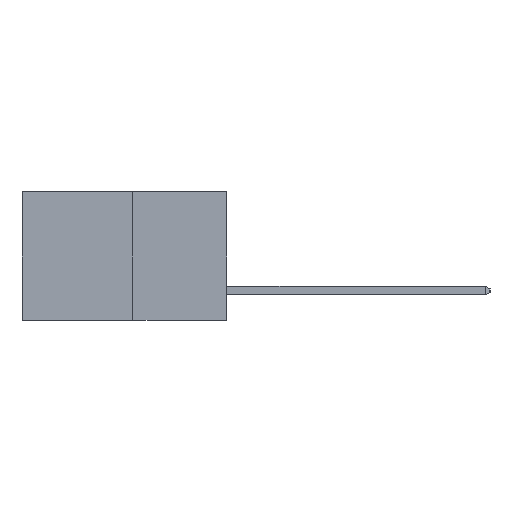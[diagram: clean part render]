
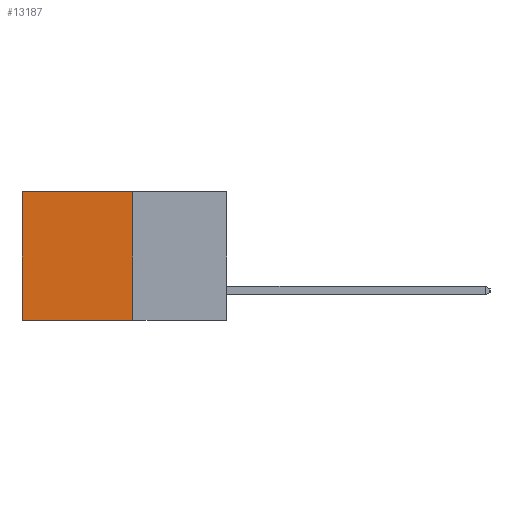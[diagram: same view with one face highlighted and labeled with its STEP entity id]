
A CAD part, left-side view. The second image highlights one B-rep face of the part: STEP entity #13187.
In plain terms, the highlighted planar face has unit normal (-1, 0, 0).
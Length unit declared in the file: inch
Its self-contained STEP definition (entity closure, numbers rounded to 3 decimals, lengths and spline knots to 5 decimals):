
#35 = CARTESIAN_POINT ( 'NONE',  ( 0.277, 0.27, -0.37 ) ) ;
#270 = PLANE ( 'NONE',  #1270 ) ;
#293 = CARTESIAN_POINT ( 'NONE',  ( 0.277, 0.59, -0.37 ) ) ;
#1270 = AXIS2_PLACEMENT_3D ( 'NONE', #7838, #8938, #2508 ) ;
#1668 = EDGE_CURVE ( 'NONE', #4268, #11095, #5689, .T. ) ;
#1980 = DIRECTION ( 'NONE',  ( 0., 1., 0. ) ) ;
#2292 = ORIENTED_EDGE ( 'NONE', *, *, #5772, .F. ) ;
#2508 = DIRECTION ( 'NONE',  ( 0., 0., -1. ) ) ;
#2675 = VECTOR ( 'NONE', #1980, 39.37008 ) ;
#3080 = DIRECTION ( 'NONE',  ( 0., 0., -1. ) ) ;
#3227 = CARTESIAN_POINT ( 'NONE',  ( 0.277, 0.27, 0. ) ) ;
#3322 = CARTESIAN_POINT ( 'NONE',  ( 0.277, 0.27, -0.37 ) ) ;
#3680 = ORIENTED_EDGE ( 'NONE', *, *, #12041, .T. ) ;
#3833 = EDGE_CURVE ( 'NONE', #4268, #5581, #13016, .T. ) ;
#4268 = VERTEX_POINT ( 'NONE', #3227 ) ;
#5500 = LINE ( 'NONE', #35, #2675 ) ;
#5581 = VERTEX_POINT ( 'NONE', #3322 ) ;
#5689 = LINE ( 'NONE', #11578, #8559 ) ;
#5772 = EDGE_CURVE ( 'NONE', #5581, #10392, #5500, .T. ) ;
#5803 = EDGE_LOOP ( 'NONE', ( #3680, #2292, #6665, #10398 ) ) ;
#6665 = ORIENTED_EDGE ( 'NONE', *, *, #3833, .F. ) ;
#7242 = VECTOR ( 'NONE', #11747, 39.37008 ) ;
#7838 = CARTESIAN_POINT ( 'NONE',  ( 0.277, 0.27, -0.37 ) ) ;
#8093 = VECTOR ( 'NONE', #3080, 39.37008 ) ;
#8444 = LINE ( 'NONE', #11714, #8093 ) ;
#8559 = VECTOR ( 'NONE', #11593, 39.37008 ) ;
#8938 = DIRECTION ( 'NONE',  ( 1., 0., 0. ) ) ;
#10392 = VERTEX_POINT ( 'NONE', #293 ) ;
#10398 = ORIENTED_EDGE ( 'NONE', *, *, #1668, .T. ) ;
#11095 = VERTEX_POINT ( 'NONE', #12380 ) ;
#11578 = CARTESIAN_POINT ( 'NONE',  ( 0.277, 0.27, 0. ) ) ;
#11593 = DIRECTION ( 'NONE',  ( 0., 1., 0. ) ) ;
#11714 = CARTESIAN_POINT ( 'NONE',  ( 0.277, 0.59, -0.37 ) ) ;
#11747 = DIRECTION ( 'NONE',  ( 0., 0., -1. ) ) ;
#11958 = CARTESIAN_POINT ( 'NONE',  ( 0.277, 0.27, -0.37 ) ) ;
#12041 = EDGE_CURVE ( 'NONE', #11095, #10392, #8444, .T. ) ;
#12380 = CARTESIAN_POINT ( 'NONE',  ( 0.277, 0.59, 0. ) ) ;
#13002 = FACE_OUTER_BOUND ( 'NONE', #5803, .T. ) ;
#13016 = LINE ( 'NONE', #11958, #7242 ) ;
#13187 = ADVANCED_FACE ( 'NONE', ( #13002 ), #270, .F. ) ;
